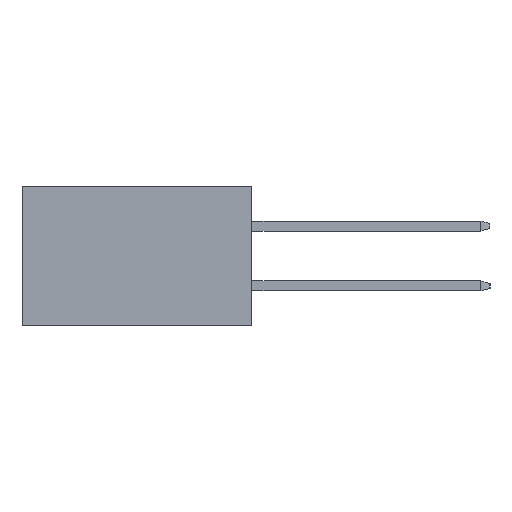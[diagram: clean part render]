
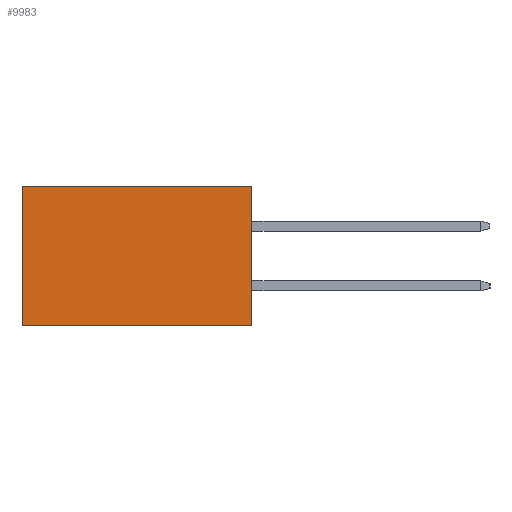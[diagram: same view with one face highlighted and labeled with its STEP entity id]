
A CAD part, left-side view. The second image highlights one B-rep face of the part: STEP entity #9983.
In plain terms, the highlighted planar face has unit normal (-1, 0, 0).
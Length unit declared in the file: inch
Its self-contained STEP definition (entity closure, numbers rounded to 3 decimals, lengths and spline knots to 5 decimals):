
#513 = CARTESIAN_POINT ( 'NONE',  ( 0.3205, 0., 0. ) ) ;
#520 = VECTOR ( 'NONE', #7419, 39.37008 ) ;
#2151 = PLANE ( 'NONE',  #2946 ) ;
#2168 = EDGE_CURVE ( 'NONE', #2866, #17321, #21229, .T. ) ;
#2240 = LINE ( 'NONE', #21694, #10170 ) ;
#2488 = CARTESIAN_POINT ( 'NONE',  ( 0.3205, 0., -0.437 ) ) ;
#2866 = VERTEX_POINT ( 'NONE', #513 ) ;
#2904 = DIRECTION ( 'NONE',  ( 0., 1., 0. ) ) ;
#2946 = AXIS2_PLACEMENT_3D ( 'NONE', #2488, #10996, #17813 ) ;
#5499 = CARTESIAN_POINT ( 'NONE',  ( 0.3205, 0.72, -0.437 ) ) ;
#5791 = FACE_OUTER_BOUND ( 'NONE', #8727, .T. ) ;
#6838 = ORIENTED_EDGE ( 'NONE', *, *, #2168, .F. ) ;
#6936 = VECTOR ( 'NONE', #2904, 39.37008 ) ;
#7392 = CARTESIAN_POINT ( 'NONE',  ( 0.3205, 0., -0.437 ) ) ;
#7419 = DIRECTION ( 'NONE',  ( 0., 0., -1. ) ) ;
#8358 = CARTESIAN_POINT ( 'NONE',  ( 0.3205, 0., -0.437 ) ) ;
#8727 = EDGE_LOOP ( 'NONE', ( #21047, #12132, #6838, #13071 ) ) ;
#9364 = CARTESIAN_POINT ( 'NONE',  ( 0.3205, 0., -0.437 ) ) ;
#9983 = ADVANCED_FACE ( 'NONE', ( #5791 ), #2151, .F. ) ;
#10126 = VECTOR ( 'NONE', #11163, 39.37008 ) ;
#10170 = VECTOR ( 'NONE', #19564, 39.37008 ) ;
#10996 = DIRECTION ( 'NONE',  ( 1., 0., 0. ) ) ;
#11163 = DIRECTION ( 'NONE',  ( 0., 0., -1. ) ) ;
#11297 = VERTEX_POINT ( 'NONE', #20427 ) ;
#11483 = EDGE_CURVE ( 'NONE', #2866, #20186, #2240, .T. ) ;
#11584 = EDGE_CURVE ( 'NONE', #17321, #11297, #16881, .T. ) ;
#12132 = ORIENTED_EDGE ( 'NONE', *, *, #11584, .F. ) ;
#13071 = ORIENTED_EDGE ( 'NONE', *, *, #11483, .T. ) ;
#15282 = EDGE_CURVE ( 'NONE', #20186, #11297, #21093, .T. ) ;
#16881 = LINE ( 'NONE', #8358, #6936 ) ;
#17321 = VERTEX_POINT ( 'NONE', #7392 ) ;
#17813 = DIRECTION ( 'NONE',  ( 0., 0., -1. ) ) ;
#18678 = CARTESIAN_POINT ( 'NONE',  ( 0.3205, 0.72, 0. ) ) ;
#19564 = DIRECTION ( 'NONE',  ( 0., 1., 0. ) ) ;
#20186 = VERTEX_POINT ( 'NONE', #18678 ) ;
#20427 = CARTESIAN_POINT ( 'NONE',  ( 0.3205, 0.72, -0.437 ) ) ;
#21047 = ORIENTED_EDGE ( 'NONE', *, *, #15282, .T. ) ;
#21093 = LINE ( 'NONE', #5499, #520 ) ;
#21229 = LINE ( 'NONE', #9364, #10126 ) ;
#21694 = CARTESIAN_POINT ( 'NONE',  ( 0.3205, 0., 0. ) ) ;
